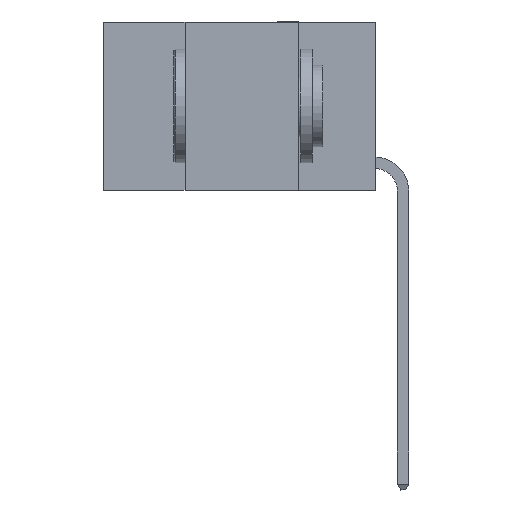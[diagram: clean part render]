
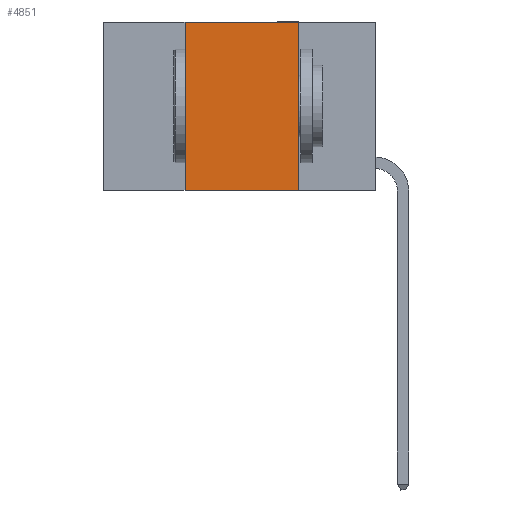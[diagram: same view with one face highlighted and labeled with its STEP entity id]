
A CAD part, left-side view. The second image highlights one B-rep face of the part: STEP entity #4851.
In plain terms, the highlighted planar face has unit normal (-1, 0, 0).
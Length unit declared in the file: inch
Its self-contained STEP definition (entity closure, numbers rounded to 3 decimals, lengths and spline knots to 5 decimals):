
#72 = CARTESIAN_POINT ( 'NONE',  ( 0., 0.42, -0.37 ) ) ;
#148 = CARTESIAN_POINT ( 'NONE',  ( 0., 0.42, 0. ) ) ;
#203 = DIRECTION ( 'NONE',  ( 1., 0., 0. ) ) ;
#334 = VECTOR ( 'NONE', #6833, 39.37008 ) ;
#1009 = VECTOR ( 'NONE', #2527, 39.37008 ) ;
#1020 = CARTESIAN_POINT ( 'NONE',  ( 0., 0.6, 0. ) ) ;
#1345 = CARTESIAN_POINT ( 'NONE',  ( 0., 0.42, 0. ) ) ;
#1355 = ORIENTED_EDGE ( 'NONE', *, *, #7883, .T. ) ;
#1411 = EDGE_LOOP ( 'NONE', ( #6952, #3912, #4993, #1355 ) ) ;
#1623 = CARTESIAN_POINT ( 'NONE',  ( 0., 0.6, 0. ) ) ;
#1881 = VERTEX_POINT ( 'NONE', #1345 ) ;
#2293 = DIRECTION ( 'NONE',  ( 0., 0., 1. ) ) ;
#2527 = DIRECTION ( 'NONE',  ( 0., -1., 0. ) ) ;
#2921 = AXIS2_PLACEMENT_3D ( 'NONE', #1623, #203, #7325 ) ;
#3666 = EDGE_CURVE ( 'NONE', #4718, #7978, #4530, .T. ) ;
#3912 = ORIENTED_EDGE ( 'NONE', *, *, #4662, .F. ) ;
#3928 = LINE ( 'NONE', #1020, #334 ) ;
#4446 = CARTESIAN_POINT ( 'NONE',  ( 0., 0.17, 0. ) ) ;
#4480 = DIRECTION ( 'NONE',  ( 0., 0., -1. ) ) ;
#4530 = LINE ( 'NONE', #4446, #4808 ) ;
#4662 = EDGE_CURVE ( 'NONE', #1881, #4718, #3928, .T. ) ;
#4718 = VERTEX_POINT ( 'NONE', #5694 ) ;
#4808 = VECTOR ( 'NONE', #4480, 39.37008 ) ;
#4851 = ADVANCED_FACE ( 'NONE', ( #5188 ), #6040, .F. ) ;
#4993 = ORIENTED_EDGE ( 'NONE', *, *, #6762, .F. ) ;
#5188 = FACE_OUTER_BOUND ( 'NONE', #1411, .T. ) ;
#5694 = CARTESIAN_POINT ( 'NONE',  ( 0., 0.17, 0. ) ) ;
#5903 = LINE ( 'NONE', #148, #8181 ) ;
#6040 = PLANE ( 'NONE',  #2921 ) ;
#6140 = CARTESIAN_POINT ( 'NONE',  ( 0., 0.6, -0.37 ) ) ;
#6391 = VERTEX_POINT ( 'NONE', #72 ) ;
#6762 = EDGE_CURVE ( 'NONE', #6391, #1881, #5903, .T. ) ;
#6833 = DIRECTION ( 'NONE',  ( 0., -1., 0. ) ) ;
#6952 = ORIENTED_EDGE ( 'NONE', *, *, #3666, .F. ) ;
#7325 = DIRECTION ( 'NONE',  ( 0., 0., -1. ) ) ;
#7826 = CARTESIAN_POINT ( 'NONE',  ( 0., 0.17, -0.37 ) ) ;
#7883 = EDGE_CURVE ( 'NONE', #6391, #7978, #9124, .T. ) ;
#7978 = VERTEX_POINT ( 'NONE', #7826 ) ;
#8181 = VECTOR ( 'NONE', #2293, 39.37008 ) ;
#9124 = LINE ( 'NONE', #6140, #1009 ) ;
